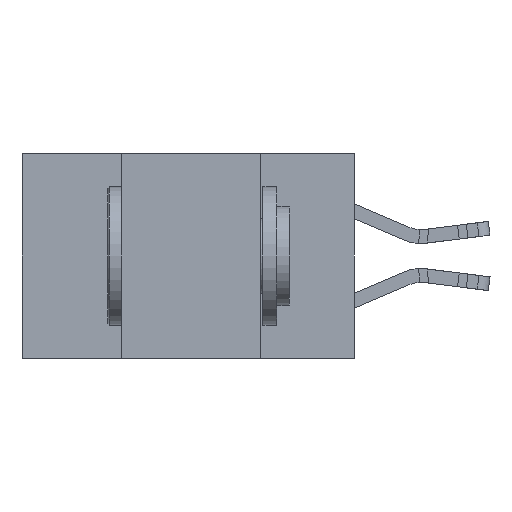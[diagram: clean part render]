
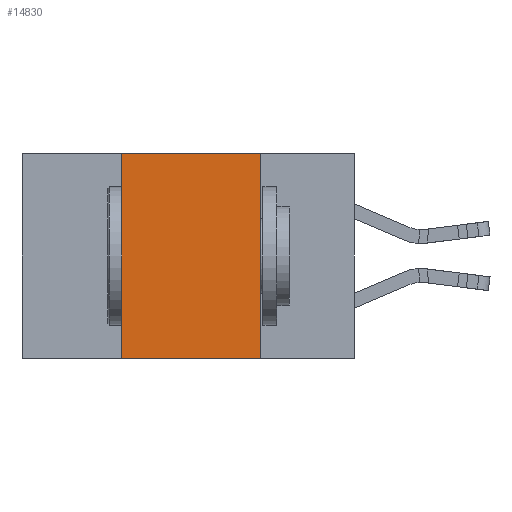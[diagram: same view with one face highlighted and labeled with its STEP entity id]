
A CAD part, left-side view. The second image highlights one B-rep face of the part: STEP entity #14830.
In plain terms, the highlighted planar face has unit normal (-1, 0, 0).
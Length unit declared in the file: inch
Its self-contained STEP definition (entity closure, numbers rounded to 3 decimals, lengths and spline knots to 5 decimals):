
#1395 = EDGE_LOOP ( 'NONE', ( #3169, #13882, #23959, #17767 ) ) ;
#2142 = VERTEX_POINT ( 'NONE', #14356 ) ;
#2371 = CARTESIAN_POINT ( 'NONE',  ( 0., 0.6, 0. ) ) ;
#2721 = LINE ( 'NONE', #2371, #7757 ) ;
#2772 = DIRECTION ( 'NONE',  ( 0., 0., -1. ) ) ;
#3169 = ORIENTED_EDGE ( 'NONE', *, *, #13084, .F. ) ;
#3645 = CARTESIAN_POINT ( 'NONE',  ( 0., 0.42, 0. ) ) ;
#4357 = VECTOR ( 'NONE', #8612, 39.37008 ) ;
#5052 = VERTEX_POINT ( 'NONE', #3645 ) ;
#6483 = DIRECTION ( 'NONE',  ( 0., 0., 1. ) ) ;
#7757 = VECTOR ( 'NONE', #15603, 39.37008 ) ;
#8612 = DIRECTION ( 'NONE',  ( 0., -1., 0. ) ) ;
#9111 = VERTEX_POINT ( 'NONE', #15895 ) ;
#9223 = EDGE_CURVE ( 'NONE', #2142, #13388, #24523, .T. ) ;
#9459 = VECTOR ( 'NONE', #15386, 39.37008 ) ;
#10446 = CARTESIAN_POINT ( 'NONE',  ( 0., 0.6, -0.37 ) ) ;
#10500 = EDGE_CURVE ( 'NONE', #2142, #5052, #20627, .T. ) ;
#11093 = VECTOR ( 'NONE', #6483, 39.37008 ) ;
#11776 = EDGE_CURVE ( 'NONE', #5052, #9111, #2721, .T. ) ;
#13084 = EDGE_CURVE ( 'NONE', #9111, #13388, #15172, .T. ) ;
#13388 = VERTEX_POINT ( 'NONE', #21241 ) ;
#13882 = ORIENTED_EDGE ( 'NONE', *, *, #11776, .F. ) ;
#14167 = DIRECTION ( 'NONE',  ( 1., 0., 0. ) ) ;
#14356 = CARTESIAN_POINT ( 'NONE',  ( 0., 0.42, -0.37 ) ) ;
#14830 = ADVANCED_FACE ( 'NONE', ( #19302 ), #19793, .F. ) ;
#15172 = LINE ( 'NONE', #21078, #9459 ) ;
#15386 = DIRECTION ( 'NONE',  ( 0., 0., -1. ) ) ;
#15603 = DIRECTION ( 'NONE',  ( 0., -1., 0. ) ) ;
#15895 = CARTESIAN_POINT ( 'NONE',  ( 0., 0.17, 0. ) ) ;
#17767 = ORIENTED_EDGE ( 'NONE', *, *, #9223, .T. ) ;
#17898 = CARTESIAN_POINT ( 'NONE',  ( 0., 0.42, -0.37 ) ) ;
#19302 = FACE_OUTER_BOUND ( 'NONE', #1395, .T. ) ;
#19793 = PLANE ( 'NONE',  #20394 ) ;
#20394 = AXIS2_PLACEMENT_3D ( 'NONE', #23599, #14167, #2772 ) ;
#20627 = LINE ( 'NONE', #17898, #11093 ) ;
#21078 = CARTESIAN_POINT ( 'NONE',  ( 0., 0.17, -0.37 ) ) ;
#21241 = CARTESIAN_POINT ( 'NONE',  ( 0., 0.17, -0.37 ) ) ;
#23599 = CARTESIAN_POINT ( 'NONE',  ( 0., 0.6, 0. ) ) ;
#23959 = ORIENTED_EDGE ( 'NONE', *, *, #10500, .F. ) ;
#24523 = LINE ( 'NONE', #10446, #4357 ) ;
